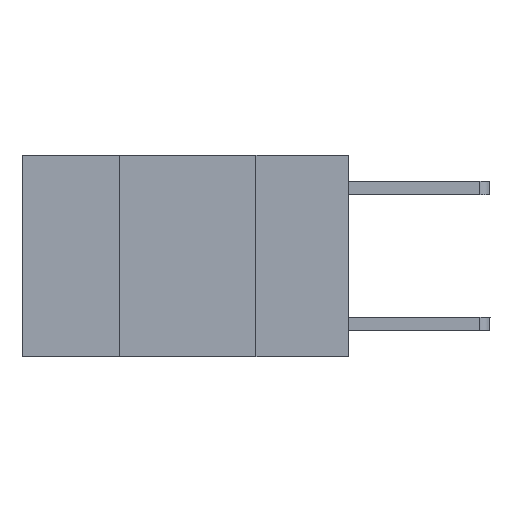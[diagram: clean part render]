
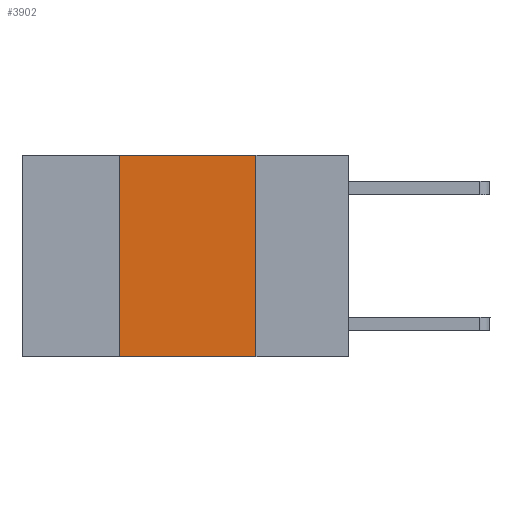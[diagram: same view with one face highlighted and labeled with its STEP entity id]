
A CAD part, left-side view. The second image highlights one B-rep face of the part: STEP entity #3902.
In plain terms, the highlighted planar face has unit normal (-1, 0, 0).
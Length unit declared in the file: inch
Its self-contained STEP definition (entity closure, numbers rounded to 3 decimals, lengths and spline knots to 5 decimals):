
#108 = ORIENTED_EDGE ( 'NONE', *, *, #7715, .F. ) ;
#199 = VECTOR ( 'NONE', #8110, 39.37008 ) ;
#1055 = DIRECTION ( 'NONE',  ( 0., 0., -1. ) ) ;
#1871 = EDGE_LOOP ( 'NONE', ( #4640, #108, #2598, #7049 ) ) ;
#1892 = DIRECTION ( 'NONE',  ( 1., 0., 0. ) ) ;
#2056 = DIRECTION ( 'NONE',  ( 0., -1., 0. ) ) ;
#2316 = CARTESIAN_POINT ( 'NONE',  ( 0., 0.42, 0. ) ) ;
#2531 = VECTOR ( 'NONE', #2056, 39.37008 ) ;
#2576 = CARTESIAN_POINT ( 'NONE',  ( 0., 0.17, -0.37 ) ) ;
#2598 = ORIENTED_EDGE ( 'NONE', *, *, #7998, .F. ) ;
#2603 = DIRECTION ( 'NONE',  ( 0., -1., 0. ) ) ;
#2752 = CARTESIAN_POINT ( 'NONE',  ( 0., 0.42, -0.37 ) ) ;
#3830 = CARTESIAN_POINT ( 'NONE',  ( 0., 0.6, 0. ) ) ;
#3896 = CARTESIAN_POINT ( 'NONE',  ( 0., 0.17, 0. ) ) ;
#3902 = ADVANCED_FACE ( 'NONE', ( #7555 ), #8464, .F. ) ;
#4017 = VERTEX_POINT ( 'NONE', #3896 ) ;
#4512 = LINE ( 'NONE', #10756, #6694 ) ;
#4528 = EDGE_CURVE ( 'NONE', #4017, #5328, #4512, .T. ) ;
#4640 = ORIENTED_EDGE ( 'NONE', *, *, #4528, .F. ) ;
#5328 = VERTEX_POINT ( 'NONE', #2576 ) ;
#5514 = LINE ( 'NONE', #8359, #9418 ) ;
#6176 = CARTESIAN_POINT ( 'NONE',  ( 0., 0.42, 0. ) ) ;
#6435 = EDGE_CURVE ( 'NONE', #9184, #5328, #5514, .T. ) ;
#6694 = VECTOR ( 'NONE', #1055, 39.37008 ) ;
#7049 = ORIENTED_EDGE ( 'NONE', *, *, #6435, .T. ) ;
#7555 = FACE_OUTER_BOUND ( 'NONE', #1871, .T. ) ;
#7711 = DIRECTION ( 'NONE',  ( 0., 0., -1. ) ) ;
#7715 = EDGE_CURVE ( 'NONE', #9201, #4017, #9040, .T. ) ;
#7991 = AXIS2_PLACEMENT_3D ( 'NONE', #10717, #1892, #7711 ) ;
#7998 = EDGE_CURVE ( 'NONE', #9184, #9201, #9160, .T. ) ;
#8110 = DIRECTION ( 'NONE',  ( 0., 0., 1. ) ) ;
#8359 = CARTESIAN_POINT ( 'NONE',  ( 0., 0.6, -0.37 ) ) ;
#8464 = PLANE ( 'NONE',  #7991 ) ;
#9040 = LINE ( 'NONE', #3830, #2531 ) ;
#9160 = LINE ( 'NONE', #2316, #199 ) ;
#9184 = VERTEX_POINT ( 'NONE', #2752 ) ;
#9201 = VERTEX_POINT ( 'NONE', #6176 ) ;
#9418 = VECTOR ( 'NONE', #2603, 39.37008 ) ;
#10717 = CARTESIAN_POINT ( 'NONE',  ( 0., 0.6, 0. ) ) ;
#10756 = CARTESIAN_POINT ( 'NONE',  ( 0., 0.17, 0. ) ) ;
